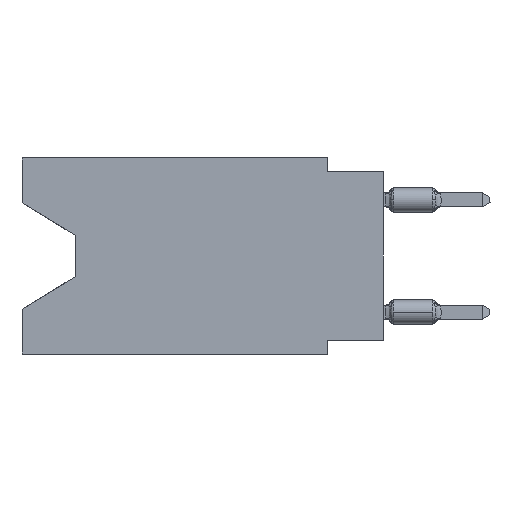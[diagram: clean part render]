
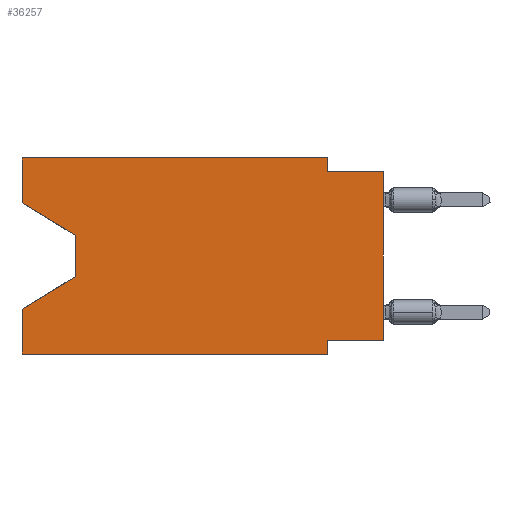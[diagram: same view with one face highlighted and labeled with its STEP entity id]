
A CAD part, left-side view. The second image highlights one B-rep face of the part: STEP entity #36257.
In plain terms, the highlighted planar face has unit normal (-1, 0, 0).
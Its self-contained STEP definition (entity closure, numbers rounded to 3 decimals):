
#180 = EDGE_CURVE ( 'NONE', #13438, #31845, #31242, .T. ) ;
#798 = ORIENTED_EDGE ( 'NONE', *, *, #7522, .T. ) ;
#907 = ORIENTED_EDGE ( 'NONE', *, *, #33074, .T. ) ;
#986 = CARTESIAN_POINT ( 'NONE',  ( 0., 16.383, 0. ) ) ;
#1143 = LINE ( 'NONE', #30536, #21387 ) ;
#1677 = VERTEX_POINT ( 'NONE', #37280 ) ;
#3704 = AXIS2_PLACEMENT_3D ( 'NONE', #35020, #14929, #32144 ) ;
#4720 = DIRECTION ( 'NONE',  ( 0., -0.855, -0.519 ) ) ;
#5075 = CARTESIAN_POINT ( 'NONE',  ( 0., 2.54, -8.89 ) ) ;
#5976 = VECTOR ( 'NONE', #37907, 1000. ) ;
#6302 = LINE ( 'NONE', #29925, #30657 ) ;
#6386 = VECTOR ( 'NONE', #4720, 1000. ) ;
#7166 = CARTESIAN_POINT ( 'NONE',  ( 0., 13.97, -5.385 ) ) ;
#7463 = CARTESIAN_POINT ( 'NONE',  ( 0., 0., 0. ) ) ;
#7522 = EDGE_CURVE ( 'NONE', #28183, #11204, #13815, .T. ) ;
#7577 = DIRECTION ( 'NONE',  ( 0., 0., -1. ) ) ;
#7839 = EDGE_CURVE ( 'NONE', #39623, #22375, #19526, .T. ) ;
#8079 = ORIENTED_EDGE ( 'NONE', *, *, #19732, .F. ) ;
#9573 = LINE ( 'NONE', #29857, #19418 ) ;
#9804 = DIRECTION ( 'NONE',  ( 0., 1., 0. ) ) ;
#10924 = LINE ( 'NONE', #31199, #6386 ) ;
#11180 = DIRECTION ( 'NONE',  ( 0., 0., 1. ) ) ;
#11204 = VERTEX_POINT ( 'NONE', #41226 ) ;
#12321 = CARTESIAN_POINT ( 'NONE',  ( 0., 13.97, -5.385 ) ) ;
#13438 = VERTEX_POINT ( 'NONE', #25124 ) ;
#13815 = LINE ( 'NONE', #7166, #22996 ) ;
#14765 = ORIENTED_EDGE ( 'NONE', *, *, #35541, .T. ) ;
#14929 = DIRECTION ( 'NONE',  ( 1., 0., 0. ) ) ;
#15568 = VERTEX_POINT ( 'NONE', #20546 ) ;
#15946 = VECTOR ( 'NONE', #19535, 1000. ) ;
#15999 = VECTOR ( 'NONE', #9804, 1000. ) ;
#16647 = CARTESIAN_POINT ( 'NONE',  ( 0., 2.54, 0. ) ) ;
#18658 = CARTESIAN_POINT ( 'NONE',  ( 0., 2.54, -8.89 ) ) ;
#19418 = VECTOR ( 'NONE', #33369, 1000. ) ;
#19494 = EDGE_LOOP ( 'NONE', ( #32421, #907, #798, #23943, #14765, #22153, #20819, #41336, #22084, #27643, #8079, #31439 ) ) ;
#19526 = LINE ( 'NONE', #23046, #15999 ) ;
#19535 = DIRECTION ( 'NONE',  ( 0., 0., -1. ) ) ;
#19732 = EDGE_CURVE ( 'NONE', #31845, #26364, #6302, .T. ) ;
#19890 = CARTESIAN_POINT ( 'NONE',  ( 0., 0., -0.635 ) ) ;
#20546 = CARTESIAN_POINT ( 'NONE',  ( 0., 16.383, -8.89 ) ) ;
#20656 = DIRECTION ( 'NONE',  ( 0., 0.855, -0.519 ) ) ;
#20819 = ORIENTED_EDGE ( 'NONE', *, *, #7839, .F. ) ;
#21387 = VECTOR ( 'NONE', #7577, 1000. ) ;
#21779 = LINE ( 'NONE', #38722, #31985 ) ;
#22084 = ORIENTED_EDGE ( 'NONE', *, *, #42999, .F. ) ;
#22153 = ORIENTED_EDGE ( 'NONE', *, *, #26692, .F. ) ;
#22375 = VERTEX_POINT ( 'NONE', #42697 ) ;
#22505 = VERTEX_POINT ( 'NONE', #43349 ) ;
#22769 = LINE ( 'NONE', #19890, #28129 ) ;
#22996 = VECTOR ( 'NONE', #20656, 1000. ) ;
#23046 = CARTESIAN_POINT ( 'NONE',  ( 0., 0., -8.255 ) ) ;
#23053 = LINE ( 'NONE', #16647, #15946 ) ;
#23943 = ORIENTED_EDGE ( 'NONE', *, *, #26532, .F. ) ;
#25124 = CARTESIAN_POINT ( 'NONE',  ( 0., 16.383, -2.038 ) ) ;
#26364 = VERTEX_POINT ( 'NONE', #28604 ) ;
#26532 = EDGE_CURVE ( 'NONE', #15568, #11204, #21779, .T. ) ;
#26692 = EDGE_CURVE ( 'NONE', #22375, #40590, #35645, .T. ) ;
#27357 = EDGE_CURVE ( 'NONE', #39623, #28406, #27755, .T. ) ;
#27484 = CARTESIAN_POINT ( 'NONE',  ( 0., 0., -0.635 ) ) ;
#27643 = ORIENTED_EDGE ( 'NONE', *, *, #29729, .F. ) ;
#27755 = LINE ( 'NONE', #7463, #5976 ) ;
#27938 = DIRECTION ( 'NONE',  ( 0., 0., 1. ) ) ;
#28129 = VECTOR ( 'NONE', #36223, 1000. ) ;
#28183 = VERTEX_POINT ( 'NONE', #12321 ) ;
#28406 = VERTEX_POINT ( 'NONE', #27484 ) ;
#28604 = CARTESIAN_POINT ( 'NONE',  ( 0., 2.54, 0. ) ) ;
#28615 = FACE_OUTER_BOUND ( 'NONE', #19494, .T. ) ;
#29729 = EDGE_CURVE ( 'NONE', #26364, #1677, #23053, .T. ) ;
#29857 = CARTESIAN_POINT ( 'NONE',  ( 0., 16.383, -8.89 ) ) ;
#29925 = CARTESIAN_POINT ( 'NONE',  ( 0., 16.383, 0. ) ) ;
#30185 = VECTOR ( 'NONE', #11180, 1000. ) ;
#30350 = EDGE_CURVE ( 'NONE', #13438, #22505, #10924, .T. ) ;
#30536 = CARTESIAN_POINT ( 'NONE',  ( 0., 13.97, -3.505 ) ) ;
#30657 = VECTOR ( 'NONE', #43389, 1000. ) ;
#31199 = CARTESIAN_POINT ( 'NONE',  ( 0., 16.383, -2.038 ) ) ;
#31242 = LINE ( 'NONE', #986, #30185 ) ;
#31439 = ORIENTED_EDGE ( 'NONE', *, *, #180, .F. ) ;
#31845 = VERTEX_POINT ( 'NONE', #40689 ) ;
#31985 = VECTOR ( 'NONE', #27938, 1000. ) ;
#32110 = DIRECTION ( 'NONE',  ( 0., 0., -1. ) ) ;
#32144 = DIRECTION ( 'NONE',  ( 0., 0., -1. ) ) ;
#32421 = ORIENTED_EDGE ( 'NONE', *, *, #30350, .T. ) ;
#33074 = EDGE_CURVE ( 'NONE', #22505, #28183, #1143, .T. ) ;
#33369 = DIRECTION ( 'NONE',  ( 0., -1., 0. ) ) ;
#35020 = CARTESIAN_POINT ( 'NONE',  ( 0., 16.383, 0. ) ) ;
#35538 = CARTESIAN_POINT ( 'NONE',  ( 0., 0., -8.255 ) ) ;
#35541 = EDGE_CURVE ( 'NONE', #15568, #40590, #9573, .T. ) ;
#35645 = LINE ( 'NONE', #18658, #38339 ) ;
#35897 = PLANE ( 'NONE',  #3704 ) ;
#36223 = DIRECTION ( 'NONE',  ( 0., -1., 0. ) ) ;
#36257 = ADVANCED_FACE ( 'NONE', ( #28615 ), #35897, .F. ) ;
#37280 = CARTESIAN_POINT ( 'NONE',  ( 0., 2.54, -0.635 ) ) ;
#37907 = DIRECTION ( 'NONE',  ( 0., 0., 1. ) ) ;
#38339 = VECTOR ( 'NONE', #32110, 1000. ) ;
#38722 = CARTESIAN_POINT ( 'NONE',  ( 0., 16.383, 0. ) ) ;
#39623 = VERTEX_POINT ( 'NONE', #35538 ) ;
#40590 = VERTEX_POINT ( 'NONE', #5075 ) ;
#40689 = CARTESIAN_POINT ( 'NONE',  ( 0., 16.383, 0. ) ) ;
#41226 = CARTESIAN_POINT ( 'NONE',  ( 0., 16.383, -6.852 ) ) ;
#41336 = ORIENTED_EDGE ( 'NONE', *, *, #27357, .T. ) ;
#42697 = CARTESIAN_POINT ( 'NONE',  ( 0., 2.54, -8.255 ) ) ;
#42999 = EDGE_CURVE ( 'NONE', #1677, #28406, #22769, .T. ) ;
#43349 = CARTESIAN_POINT ( 'NONE',  ( 0., 13.97, -3.505 ) ) ;
#43389 = DIRECTION ( 'NONE',  ( 0., -1., 0. ) ) ;
